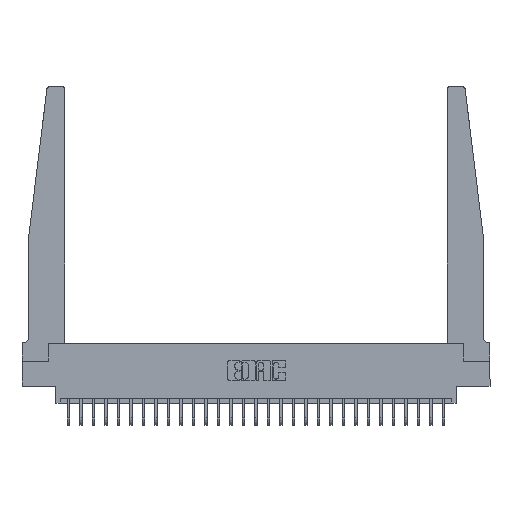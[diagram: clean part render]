
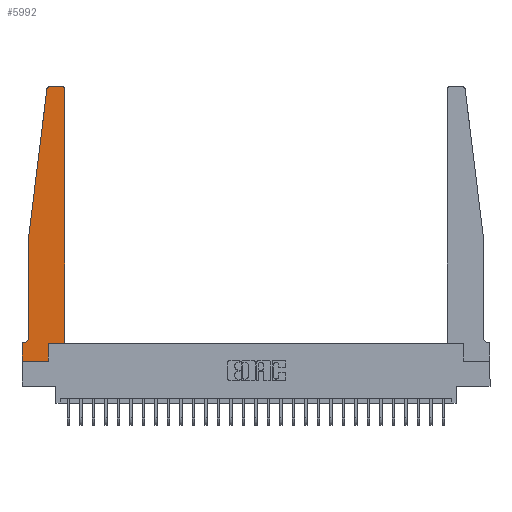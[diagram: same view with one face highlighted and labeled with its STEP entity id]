
A CAD part, top view. The second image highlights one B-rep face of the part: STEP entity #5992.
In plain terms, the highlighted planar face has unit normal (0, 0, 1).
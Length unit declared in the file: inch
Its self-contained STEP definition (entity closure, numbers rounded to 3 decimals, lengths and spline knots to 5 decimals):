
#193 = CARTESIAN_POINT ( 'NONE',  ( 0.395, 2.75, 0.37 ) ) ;
#534 = CARTESIAN_POINT ( 'NONE',  ( 0.065, 0.2375, 0.37 ) ) ;
#587 = EDGE_CURVE ( 'NONE', #17756, #5824, #10529, .T. ) ;
#866 = VECTOR ( 'NONE', #20815, 39.37008 ) ;
#1166 = VECTOR ( 'NONE', #24395, 39.37008 ) ;
#1253 = VERTEX_POINT ( 'NONE', #8346 ) ;
#1266 = EDGE_LOOP ( 'NONE', ( #21502, #21806, #27438, #7919, #25338, #7337, #4375, #7941, #21206, #18461, #6959, #24653 ) ) ;
#1854 = CARTESIAN_POINT ( 'NONE',  ( 0.065, 1.25, 0.37 ) ) ;
#2093 = EDGE_CURVE ( 'NONE', #1253, #12015, #22188, .T. ) ;
#2301 = EDGE_CURVE ( 'NONE', #7188, #17920, #17015, .T. ) ;
#3053 = VECTOR ( 'NONE', #20211, 39.37008 ) ;
#3167 = EDGE_CURVE ( 'NONE', #3782, #16783, #24125, .T. ) ;
#3782 = VERTEX_POINT ( 'NONE', #8938 ) ;
#4098 = CIRCLE ( 'NONE', #11723, 0.05 ) ;
#4180 = EDGE_CURVE ( 'NONE', #12000, #18338, #27688, .T. ) ;
#4311 = PLANE ( 'NONE',  #9297 ) ;
#4375 = ORIENTED_EDGE ( 'NONE', *, *, #3167, .T. ) ;
#4797 = CARTESIAN_POINT ( 'NONE',  ( 0.2605, 0.18, 0.37 ) ) ;
#5824 = VERTEX_POINT ( 'NONE', #8267 ) ;
#5992 = ADVANCED_FACE ( 'NONE', ( #23062 ), #4311, .T. ) ;
#6959 = ORIENTED_EDGE ( 'NONE', *, *, #2301, .T. ) ;
#7140 = CARTESIAN_POINT ( 'NONE',  ( 0.015, 0.1875, 0.37 ) ) ;
#7143 = CARTESIAN_POINT ( 'NONE',  ( 0.065, 1.25, 0.37 ) ) ;
#7188 = VERTEX_POINT ( 'NONE', #26622 ) ;
#7232 = CARTESIAN_POINT ( 'NONE',  ( 0.425, 2.72, 0.37 ) ) ;
#7306 = EDGE_CURVE ( 'NONE', #16783, #1253, #14383, .T. ) ;
#7337 = ORIENTED_EDGE ( 'NONE', *, *, #22801, .T. ) ;
#7452 = LINE ( 'NONE', #1854, #866 ) ;
#7882 = EDGE_CURVE ( 'NONE', #5824, #27585, #20136, .T. ) ;
#7919 = ORIENTED_EDGE ( 'NONE', *, *, #4180, .T. ) ;
#7941 = ORIENTED_EDGE ( 'NONE', *, *, #7306, .T. ) ;
#8267 = CARTESIAN_POINT ( 'NONE',  ( 0.27653, 2.75, 0.37 ) ) ;
#8294 = EDGE_CURVE ( 'NONE', #17920, #17756, #17313, .T. ) ;
#8346 = CARTESIAN_POINT ( 'NONE',  ( 0.2605, 0., 0.37 ) ) ;
#8653 = CARTESIAN_POINT ( 'NONE',  ( 0., 0.1875, 0.37 ) ) ;
#8810 = VECTOR ( 'NONE', #13069, 39.37008 ) ;
#8938 = CARTESIAN_POINT ( 'NONE',  ( 0., 0.1875, 0.37 ) ) ;
#9103 = VECTOR ( 'NONE', #9228, 39.37008 ) ;
#9228 = DIRECTION ( 'NONE',  ( 0., 1., 0. ) ) ;
#9297 = AXIS2_PLACEMENT_3D ( 'NONE', #8653, #15209, #26379 ) ;
#9519 = DIRECTION ( 'NONE',  ( 0., 0., 1. ) ) ;
#10529 = LINE ( 'NONE', #23167, #27311 ) ;
#10830 = DIRECTION ( 'NONE',  ( 0., 1., 0. ) ) ;
#10886 = VERTEX_POINT ( 'NONE', #7140 ) ;
#11566 = VECTOR ( 'NONE', #10830, 39.37008 ) ;
#11723 = AXIS2_PLACEMENT_3D ( 'NONE', #13444, #13534, #15733 ) ;
#11778 = DIRECTION ( 'NONE',  ( 1., 0., 0. ) ) ;
#12000 = VERTEX_POINT ( 'NONE', #7143 ) ;
#12015 = VERTEX_POINT ( 'NONE', #25680 ) ;
#12953 = CARTESIAN_POINT ( 'NONE',  ( 0.425, 0.18, 0.37 ) ) ;
#13069 = DIRECTION ( 'NONE',  ( 0., -1., 0. ) ) ;
#13444 = CARTESIAN_POINT ( 'NONE',  ( 0.015, 0.2375, 0.37 ) ) ;
#13534 = DIRECTION ( 'NONE',  ( 0., 0., -1. ) ) ;
#14383 = LINE ( 'NONE', #25424, #27378 ) ;
#15209 = DIRECTION ( 'NONE',  ( 0., 0., 1. ) ) ;
#15228 = EDGE_CURVE ( 'NONE', #18338, #10886, #4098, .T. ) ;
#15733 = DIRECTION ( 'NONE',  ( -1., 0., 0. ) ) ;
#16226 = CARTESIAN_POINT ( 'NONE',  ( 0.24675, 2.72367, 0.37 ) ) ;
#16574 = EDGE_CURVE ( 'NONE', #12015, #7188, #17475, .T. ) ;
#16686 = CARTESIAN_POINT ( 'NONE',  ( 0., 0., 0.37 ) ) ;
#16742 = AXIS2_PLACEMENT_3D ( 'NONE', #27661, #27766, #27473 ) ;
#16783 = VERTEX_POINT ( 'NONE', #16686 ) ;
#16784 = DIRECTION ( 'NONE',  ( -1., 0., 0. ) ) ;
#17015 = LINE ( 'NONE', #12953, #11566 ) ;
#17188 = DIRECTION ( 'NONE',  ( 1., 0., 0. ) ) ;
#17313 = CIRCLE ( 'NONE', #18745, 0.03 ) ;
#17475 = LINE ( 'NONE', #18096, #3053 ) ;
#17756 = VERTEX_POINT ( 'NONE', #193 ) ;
#17920 = VERTEX_POINT ( 'NONE', #7232 ) ;
#18096 = CARTESIAN_POINT ( 'NONE',  ( 0.425, 0.18, 0.37 ) ) ;
#18338 = VERTEX_POINT ( 'NONE', #534 ) ;
#18461 = ORIENTED_EDGE ( 'NONE', *, *, #16574, .T. ) ;
#18745 = AXIS2_PLACEMENT_3D ( 'NONE', #22676, #9519, #11778 ) ;
#19001 = VECTOR ( 'NONE', #24355, 39.37008 ) ;
#20136 = CIRCLE ( 'NONE', #16742, 0.03 ) ;
#20211 = DIRECTION ( 'NONE',  ( 1., 0., 0. ) ) ;
#20457 = CARTESIAN_POINT ( 'NONE',  ( 0., 0., 0.37 ) ) ;
#20815 = DIRECTION ( 'NONE',  ( -0.122, -0.992, 0. ) ) ;
#20821 = LINE ( 'NONE', #26595, #1166 ) ;
#21206 = ORIENTED_EDGE ( 'NONE', *, *, #2093, .T. ) ;
#21502 = ORIENTED_EDGE ( 'NONE', *, *, #587, .T. ) ;
#21806 = ORIENTED_EDGE ( 'NONE', *, *, #7882, .T. ) ;
#21981 = EDGE_CURVE ( 'NONE', #27585, #12000, #7452, .T. ) ;
#22188 = LINE ( 'NONE', #4797, #9103 ) ;
#22676 = CARTESIAN_POINT ( 'NONE',  ( 0.395, 2.72, 0.37 ) ) ;
#22801 = EDGE_CURVE ( 'NONE', #10886, #3782, #20821, .T. ) ;
#23062 = FACE_OUTER_BOUND ( 'NONE', #1266, .T. ) ;
#23167 = CARTESIAN_POINT ( 'NONE',  ( 0.25, 2.75, 0.37 ) ) ;
#23974 = CARTESIAN_POINT ( 'NONE',  ( 0.065, 1.25, 0.37 ) ) ;
#24125 = LINE ( 'NONE', #20457, #19001 ) ;
#24355 = DIRECTION ( 'NONE',  ( 0., -1., 0. ) ) ;
#24395 = DIRECTION ( 'NONE',  ( -1., 0., 0. ) ) ;
#24653 = ORIENTED_EDGE ( 'NONE', *, *, #8294, .T. ) ;
#25338 = ORIENTED_EDGE ( 'NONE', *, *, #15228, .T. ) ;
#25424 = CARTESIAN_POINT ( 'NONE',  ( 0., 0., 0.37 ) ) ;
#25680 = CARTESIAN_POINT ( 'NONE',  ( 0.2605, 0.18, 0.37 ) ) ;
#26379 = DIRECTION ( 'NONE',  ( 1., 0., 0. ) ) ;
#26595 = CARTESIAN_POINT ( 'NONE',  ( 0.065, 0.1875, 0.37 ) ) ;
#26622 = CARTESIAN_POINT ( 'NONE',  ( 0.425, 0.18, 0.37 ) ) ;
#27311 = VECTOR ( 'NONE', #16784, 39.37008 ) ;
#27378 = VECTOR ( 'NONE', #17188, 39.37008 ) ;
#27438 = ORIENTED_EDGE ( 'NONE', *, *, #21981, .T. ) ;
#27473 = DIRECTION ( 'NONE',  ( 1., 0., 0. ) ) ;
#27585 = VERTEX_POINT ( 'NONE', #16226 ) ;
#27661 = CARTESIAN_POINT ( 'NONE',  ( 0.27653, 2.72, 0.37 ) ) ;
#27688 = LINE ( 'NONE', #23974, #8810 ) ;
#27766 = DIRECTION ( 'NONE',  ( 0., 0., 1. ) ) ;
